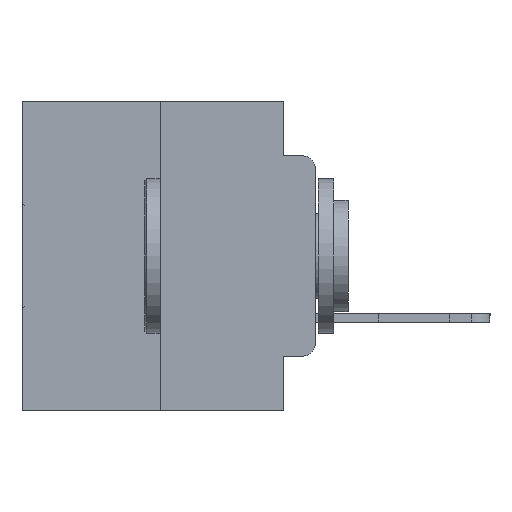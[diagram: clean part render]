
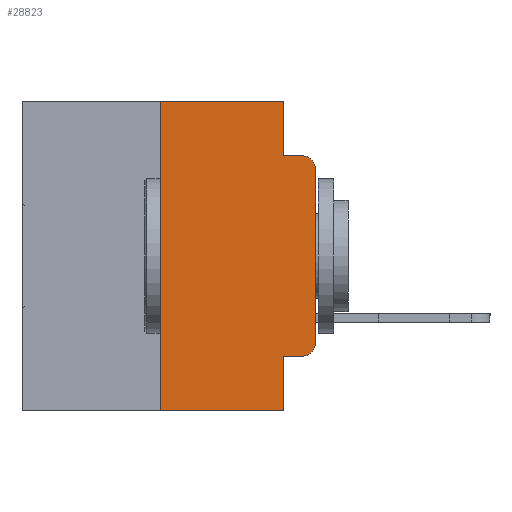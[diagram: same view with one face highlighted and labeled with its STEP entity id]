
A CAD part, left-side view. The second image highlights one B-rep face of the part: STEP entity #28823.
In plain terms, the highlighted planar face has unit normal (-1, 0, 0).
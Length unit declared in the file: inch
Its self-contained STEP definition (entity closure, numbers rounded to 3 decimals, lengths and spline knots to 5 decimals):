
#141 = EDGE_CURVE ( 'NONE', #494, #23336, #14713, .T. ) ;
#233 = DIRECTION ( 'NONE',  ( -1., 0., 0. ) ) ;
#338 = CIRCLE ( 'NONE', #8613, 0.02 ) ;
#494 = VERTEX_POINT ( 'NONE', #3298 ) ;
#628 = CARTESIAN_POINT ( 'NONE',  ( 0., 0.051, -0.5 ) ) ;
#1383 = CARTESIAN_POINT ( 'NONE',  ( 0., 0.25, 0. ) ) ;
#3298 = CARTESIAN_POINT ( 'NONE',  ( 0., 0.051, -0.4115 ) ) ;
#3308 = EDGE_CURVE ( 'NONE', #23221, #9626, #13081, .T. ) ;
#3844 = CARTESIAN_POINT ( 'NONE',  ( 0., 0.051, -0.0885 ) ) ;
#4631 = ORIENTED_EDGE ( 'NONE', *, *, #17271, .F. ) ;
#4877 = EDGE_CURVE ( 'NONE', #9057, #23523, #6368, .T. ) ;
#4985 = VERTEX_POINT ( 'NONE', #17132 ) ;
#6368 = LINE ( 'NONE', #7334, #24235 ) ;
#6696 = CIRCLE ( 'NONE', #14396, 0.02 ) ;
#6837 = VECTOR ( 'NONE', #29294, 39.37008 ) ;
#6930 = CARTESIAN_POINT ( 'NONE',  ( 0., 0.473, 0. ) ) ;
#7334 = CARTESIAN_POINT ( 'NONE',  ( 0., 0.051, 0. ) ) ;
#7352 = DIRECTION ( 'NONE',  ( 0., -1., 0. ) ) ;
#7580 = ORIENTED_EDGE ( 'NONE', *, *, #28848, .T. ) ;
#7810 = VECTOR ( 'NONE', #13196, 39.37008 ) ;
#7950 = CARTESIAN_POINT ( 'NONE',  ( 0., 0., 0. ) ) ;
#8489 = VECTOR ( 'NONE', #20537, 39.37008 ) ;
#8613 = AXIS2_PLACEMENT_3D ( 'NONE', #14291, #233, #16638 ) ;
#8692 = CARTESIAN_POINT ( 'NONE',  ( 0., 0.25, 0. ) ) ;
#9057 = VERTEX_POINT ( 'NONE', #18101 ) ;
#9295 = DIRECTION ( 'NONE',  ( 1., 0., 0. ) ) ;
#9402 = ORIENTED_EDGE ( 'NONE', *, *, #11185, .T. ) ;
#9601 = EDGE_CURVE ( 'NONE', #23523, #28639, #14032, .T. ) ;
#9626 = VERTEX_POINT ( 'NONE', #8692 ) ;
#9972 = AXIS2_PLACEMENT_3D ( 'NONE', #6930, #9295, #25551 ) ;
#10871 = LINE ( 'NONE', #12074, #16315 ) ;
#11185 = EDGE_CURVE ( 'NONE', #21546, #28639, #338, .T. ) ;
#11702 = FACE_OUTER_BOUND ( 'NONE', #15394, .T. ) ;
#12074 = CARTESIAN_POINT ( 'NONE',  ( 0., 0.473, -0.5 ) ) ;
#12121 = DIRECTION ( 'NONE',  ( -1., 0., 0. ) ) ;
#12342 = ORIENTED_EDGE ( 'NONE', *, *, #17446, .T. ) ;
#12726 = EDGE_CURVE ( 'NONE', #4985, #21546, #22541, .T. ) ;
#13081 = LINE ( 'NONE', #1383, #6837 ) ;
#13196 = DIRECTION ( 'NONE',  ( 0., -1., 0. ) ) ;
#13307 = VERTEX_POINT ( 'NONE', #29042 ) ;
#13392 = CARTESIAN_POINT ( 'NONE',  ( 0., 0.051, 0. ) ) ;
#13719 = CARTESIAN_POINT ( 'NONE',  ( 0., 0.473, 0. ) ) ;
#14032 = LINE ( 'NONE', #24755, #7810 ) ;
#14291 = CARTESIAN_POINT ( 'NONE',  ( 0., 0.02, -0.1085 ) ) ;
#14396 = AXIS2_PLACEMENT_3D ( 'NONE', #26024, #12121, #28328 ) ;
#14713 = LINE ( 'NONE', #13392, #8489 ) ;
#15294 = CARTESIAN_POINT ( 'NONE',  ( 0., 0., -0.1085 ) ) ;
#15394 = EDGE_LOOP ( 'NONE', ( #21072, #9402, #22515, #28651, #4631, #17791, #12342, #24693, #7580, #26136 ) ) ;
#15643 = CARTESIAN_POINT ( 'NONE',  ( 0., 0.02, -0.0885 ) ) ;
#16315 = VECTOR ( 'NONE', #7352, 39.37008 ) ;
#16415 = VECTOR ( 'NONE', #25663, 39.37008 ) ;
#16638 = DIRECTION ( 'NONE',  ( 0., 0., -1. ) ) ;
#16694 = LINE ( 'NONE', #13719, #21418 ) ;
#17132 = CARTESIAN_POINT ( 'NONE',  ( 0., 0., -0.3915 ) ) ;
#17151 = LINE ( 'NONE', #23328, #16415 ) ;
#17271 = EDGE_CURVE ( 'NONE', #9626, #9057, #16694, .T. ) ;
#17446 = EDGE_CURVE ( 'NONE', #23221, #23336, #10871, .T. ) ;
#17791 = ORIENTED_EDGE ( 'NONE', *, *, #3308, .F. ) ;
#18101 = CARTESIAN_POINT ( 'NONE',  ( 0., 0.051, 0. ) ) ;
#20537 = DIRECTION ( 'NONE',  ( 0., 0., -1. ) ) ;
#20912 = PLANE ( 'NONE',  #9972 ) ;
#21072 = ORIENTED_EDGE ( 'NONE', *, *, #12726, .T. ) ;
#21418 = VECTOR ( 'NONE', #27601, 39.37008 ) ;
#21546 = VERTEX_POINT ( 'NONE', #15294 ) ;
#21805 = DIRECTION ( 'NONE',  ( 0., 0., 1. ) ) ;
#22515 = ORIENTED_EDGE ( 'NONE', *, *, #9601, .F. ) ;
#22541 = LINE ( 'NONE', #7950, #27948 ) ;
#23221 = VERTEX_POINT ( 'NONE', #28153 ) ;
#23328 = CARTESIAN_POINT ( 'NONE',  ( 0., 0.051, -0.4115 ) ) ;
#23336 = VERTEX_POINT ( 'NONE', #628 ) ;
#23523 = VERTEX_POINT ( 'NONE', #3844 ) ;
#23618 = DIRECTION ( 'NONE',  ( 0., 0., -1. ) ) ;
#24235 = VECTOR ( 'NONE', #23618, 39.37008 ) ;
#24693 = ORIENTED_EDGE ( 'NONE', *, *, #141, .F. ) ;
#24755 = CARTESIAN_POINT ( 'NONE',  ( 0., 0.051, -0.0885 ) ) ;
#25551 = DIRECTION ( 'NONE',  ( 0., 0., -1. ) ) ;
#25663 = DIRECTION ( 'NONE',  ( 0., -1., 0. ) ) ;
#25757 = EDGE_CURVE ( 'NONE', #13307, #4985, #6696, .T. ) ;
#26024 = CARTESIAN_POINT ( 'NONE',  ( 0., 0.02, -0.3915 ) ) ;
#26136 = ORIENTED_EDGE ( 'NONE', *, *, #25757, .T. ) ;
#27601 = DIRECTION ( 'NONE',  ( 0., -1., 0. ) ) ;
#27948 = VECTOR ( 'NONE', #21805, 39.37008 ) ;
#28153 = CARTESIAN_POINT ( 'NONE',  ( 0., 0.25, -0.5 ) ) ;
#28328 = DIRECTION ( 'NONE',  ( 0., 0., -1. ) ) ;
#28639 = VERTEX_POINT ( 'NONE', #15643 ) ;
#28651 = ORIENTED_EDGE ( 'NONE', *, *, #4877, .F. ) ;
#28823 = ADVANCED_FACE ( 'NONE', ( #11702 ), #20912, .F. ) ;
#28848 = EDGE_CURVE ( 'NONE', #494, #13307, #17151, .T. ) ;
#29042 = CARTESIAN_POINT ( 'NONE',  ( 0., 0.02, -0.4115 ) ) ;
#29294 = DIRECTION ( 'NONE',  ( 0., 0., 1. ) ) ;
